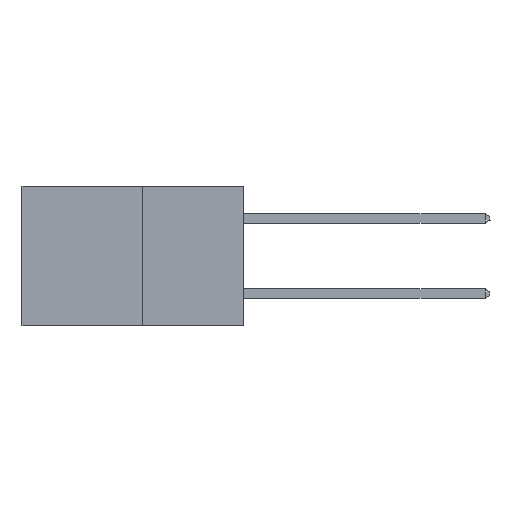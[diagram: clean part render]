
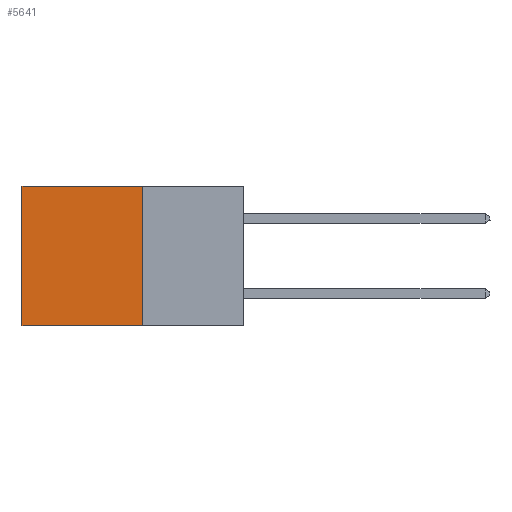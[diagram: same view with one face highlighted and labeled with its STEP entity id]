
A CAD part, left-side view. The second image highlights one B-rep face of the part: STEP entity #5641.
In plain terms, the highlighted planar face has unit normal (-1, 0, 0).
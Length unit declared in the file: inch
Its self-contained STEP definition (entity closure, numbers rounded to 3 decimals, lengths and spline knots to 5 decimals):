
#175 = DIRECTION ( 'NONE',  ( 1., 0., 0. ) ) ;
#539 = VECTOR ( 'NONE', #9388, 39.37008 ) ;
#577 = ORIENTED_EDGE ( 'NONE', *, *, #8903, .F. ) ;
#1091 = LINE ( 'NONE', #8328, #4617 ) ;
#1413 = ORIENTED_EDGE ( 'NONE', *, *, #2164, .T. ) ;
#1667 = LINE ( 'NONE', #5197, #5635 ) ;
#2164 = EDGE_CURVE ( 'NONE', #4336, #2641, #4498, .T. ) ;
#2243 = ORIENTED_EDGE ( 'NONE', *, *, #2393, .T. ) ;
#2393 = EDGE_CURVE ( 'NONE', #8263, #4336, #1091, .T. ) ;
#2617 = LINE ( 'NONE', #7974, #539 ) ;
#2641 = VERTEX_POINT ( 'NONE', #9601 ) ;
#3050 = DIRECTION ( 'NONE',  ( 0., 0., -1. ) ) ;
#4336 = VERTEX_POINT ( 'NONE', #5182 ) ;
#4498 = LINE ( 'NONE', #7120, #8644 ) ;
#4617 = VECTOR ( 'NONE', #8458, 39.37008 ) ;
#4682 = CARTESIAN_POINT ( 'NONE',  ( 0.277, 0.27, -0.37 ) ) ;
#5182 = CARTESIAN_POINT ( 'NONE',  ( 0.277, 0.59, 0. ) ) ;
#5197 = CARTESIAN_POINT ( 'NONE',  ( 0.277, 0.27, -0.37 ) ) ;
#5281 = CARTESIAN_POINT ( 'NONE',  ( 0.277, 0.27, -0.37 ) ) ;
#5399 = ORIENTED_EDGE ( 'NONE', *, *, #7711, .F. ) ;
#5439 = DIRECTION ( 'NONE',  ( 0., 0., -1. ) ) ;
#5635 = VECTOR ( 'NONE', #5976, 39.37008 ) ;
#5641 = ADVANCED_FACE ( 'NONE', ( #9372 ), #8362, .F. ) ;
#5976 = DIRECTION ( 'NONE',  ( 0., 0., -1. ) ) ;
#7099 = VERTEX_POINT ( 'NONE', #5281 ) ;
#7120 = CARTESIAN_POINT ( 'NONE',  ( 0.277, 0.59, -0.37 ) ) ;
#7711 = EDGE_CURVE ( 'NONE', #8263, #7099, #1667, .T. ) ;
#7974 = CARTESIAN_POINT ( 'NONE',  ( 0.277, 0.27, -0.37 ) ) ;
#8263 = VERTEX_POINT ( 'NONE', #9428 ) ;
#8328 = CARTESIAN_POINT ( 'NONE',  ( 0.277, 0.27, 0. ) ) ;
#8362 = PLANE ( 'NONE',  #8446 ) ;
#8446 = AXIS2_PLACEMENT_3D ( 'NONE', #4682, #175, #5439 ) ;
#8458 = DIRECTION ( 'NONE',  ( 0., 1., 0. ) ) ;
#8644 = VECTOR ( 'NONE', #3050, 39.37008 ) ;
#8772 = EDGE_LOOP ( 'NONE', ( #1413, #577, #5399, #2243 ) ) ;
#8903 = EDGE_CURVE ( 'NONE', #7099, #2641, #2617, .T. ) ;
#9372 = FACE_OUTER_BOUND ( 'NONE', #8772, .T. ) ;
#9388 = DIRECTION ( 'NONE',  ( 0., 1., 0. ) ) ;
#9428 = CARTESIAN_POINT ( 'NONE',  ( 0.277, 0.27, 0. ) ) ;
#9601 = CARTESIAN_POINT ( 'NONE',  ( 0.277, 0.59, -0.37 ) ) ;
